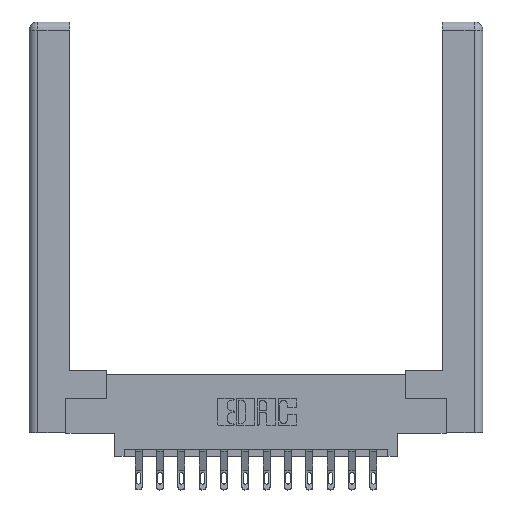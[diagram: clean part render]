
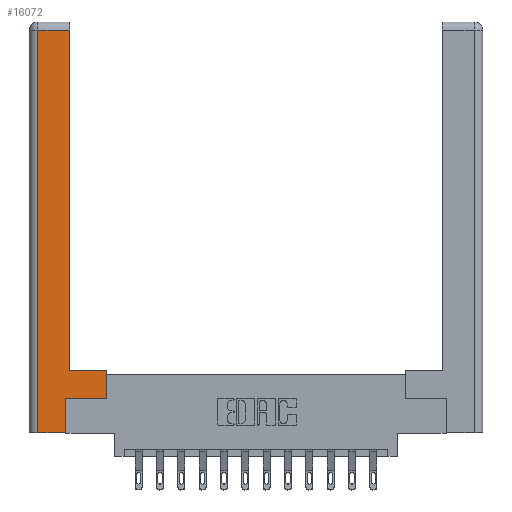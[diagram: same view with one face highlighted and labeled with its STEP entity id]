
A CAD part, top view. The second image highlights one B-rep face of the part: STEP entity #16072.
In plain terms, the highlighted planar face has unit normal (0, 0, 1).
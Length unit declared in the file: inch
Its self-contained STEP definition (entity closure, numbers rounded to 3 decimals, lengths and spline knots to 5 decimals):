
#4 = VERTEX_POINT ( 'NONE', #5458 ) ;
#204 = CARTESIAN_POINT ( 'NONE',  ( 0.0615, 0., 0. ) ) ;
#769 = EDGE_CURVE ( 'NONE', #12303, #15962, #13163, .T. ) ;
#890 = CARTESIAN_POINT ( 'NONE',  ( 0., 0., 0. ) ) ;
#1035 = VECTOR ( 'NONE', #10809, 39.37008 ) ;
#1246 = VECTOR ( 'NONE', #10216, 39.37008 ) ;
#1797 = CARTESIAN_POINT ( 'NONE',  ( 0.295, 2.94, 0. ) ) ;
#2032 = DIRECTION ( 'NONE',  ( 1., 0., 0. ) ) ;
#2476 = LINE ( 'NONE', #3857, #11309 ) ;
#3183 = ORIENTED_EDGE ( 'NONE', *, *, #4606, .T. ) ;
#3334 = ORIENTED_EDGE ( 'NONE', *, *, #7409, .T. ) ;
#3857 = CARTESIAN_POINT ( 'NONE',  ( 0.0615, 2.94, 0. ) ) ;
#3970 = CARTESIAN_POINT ( 'NONE',  ( 0.0615, 0., 0. ) ) ;
#4220 = VERTEX_POINT ( 'NONE', #6831 ) ;
#4551 = LINE ( 'NONE', #5077, #1246 ) ;
#4606 = EDGE_CURVE ( 'NONE', #12475, #7044, #2476, .T. ) ;
#4971 = DIRECTION ( 'NONE',  ( -1., 0., 0. ) ) ;
#5054 = CARTESIAN_POINT ( 'NONE',  ( 0.0615, 2.94, 0. ) ) ;
#5077 = CARTESIAN_POINT ( 'NONE',  ( 0.565, 0.45, 0. ) ) ;
#5188 = DIRECTION ( 'NONE',  ( 0., -1., 0. ) ) ;
#5458 = CARTESIAN_POINT ( 'NONE',  ( 0.565, 0.245, 0. ) ) ;
#5678 = AXIS2_PLACEMENT_3D ( 'NONE', #890, #9461, #12070 ) ;
#5933 = EDGE_CURVE ( 'NONE', #4220, #4, #11906, .T. ) ;
#6303 = CARTESIAN_POINT ( 'NONE',  ( 0.295, 0.45, 0. ) ) ;
#6445 = EDGE_CURVE ( 'NONE', #15962, #4220, #7293, .T. ) ;
#6590 = EDGE_LOOP ( 'NONE', ( #13713, #3183, #12075, #7782, #12550, #9775, #11407, #3334 ) ) ;
#6817 = VECTOR ( 'NONE', #2032, 39.37008 ) ;
#6831 = CARTESIAN_POINT ( 'NONE',  ( 0.265, 0.245, 0. ) ) ;
#6881 = CARTESIAN_POINT ( 'NONE',  ( 0.565, 0.45, 0. ) ) ;
#7044 = VERTEX_POINT ( 'NONE', #5054 ) ;
#7067 = PLANE ( 'NONE',  #5678 ) ;
#7175 = CARTESIAN_POINT ( 'NONE',  ( 0.295, 3., 0. ) ) ;
#7215 = VERTEX_POINT ( 'NONE', #8296 ) ;
#7276 = EDGE_CURVE ( 'NONE', #7215, #12475, #15420, .T. ) ;
#7293 = LINE ( 'NONE', #9532, #1035 ) ;
#7409 = EDGE_CURVE ( 'NONE', #12609, #7215, #15790, .T. ) ;
#7497 = LINE ( 'NONE', #204, #13440 ) ;
#7782 = ORIENTED_EDGE ( 'NONE', *, *, #769, .T. ) ;
#8262 = CARTESIAN_POINT ( 'NONE',  ( 0.265, 0., 0. ) ) ;
#8272 = VECTOR ( 'NONE', #8462, 39.37008 ) ;
#8296 = CARTESIAN_POINT ( 'NONE',  ( 0.295, 0.45, 0. ) ) ;
#8462 = DIRECTION ( 'NONE',  ( 0., 1., 0. ) ) ;
#8713 = VECTOR ( 'NONE', #12404, 39.37008 ) ;
#9461 = DIRECTION ( 'NONE',  ( 0., 0., -1. ) ) ;
#9532 = CARTESIAN_POINT ( 'NONE',  ( 0.265, 0.245, 0. ) ) ;
#9775 = ORIENTED_EDGE ( 'NONE', *, *, #5933, .T. ) ;
#10216 = DIRECTION ( 'NONE',  ( 0., 1., 0. ) ) ;
#10809 = DIRECTION ( 'NONE',  ( 0., 1., 0. ) ) ;
#11309 = VECTOR ( 'NONE', #11817, 39.37008 ) ;
#11407 = ORIENTED_EDGE ( 'NONE', *, *, #14374, .T. ) ;
#11817 = DIRECTION ( 'NONE',  ( -1., 0., 0. ) ) ;
#11906 = LINE ( 'NONE', #13725, #8713 ) ;
#12070 = DIRECTION ( 'NONE',  ( -1., 0., 0. ) ) ;
#12075 = ORIENTED_EDGE ( 'NONE', *, *, #14395, .T. ) ;
#12303 = VERTEX_POINT ( 'NONE', #3970 ) ;
#12404 = DIRECTION ( 'NONE',  ( 1., 0., 0. ) ) ;
#12429 = VECTOR ( 'NONE', #4971, 39.37008 ) ;
#12475 = VERTEX_POINT ( 'NONE', #1797 ) ;
#12550 = ORIENTED_EDGE ( 'NONE', *, *, #6445, .T. ) ;
#12609 = VERTEX_POINT ( 'NONE', #6881 ) ;
#12764 = FACE_OUTER_BOUND ( 'NONE', #6590, .T. ) ;
#13163 = LINE ( 'NONE', #8262, #6817 ) ;
#13440 = VECTOR ( 'NONE', #5188, 39.37008 ) ;
#13713 = ORIENTED_EDGE ( 'NONE', *, *, #7276, .T. ) ;
#13725 = CARTESIAN_POINT ( 'NONE',  ( 0.565, 0.245, 0. ) ) ;
#14005 = CARTESIAN_POINT ( 'NONE',  ( 0.265, 0., 0. ) ) ;
#14374 = EDGE_CURVE ( 'NONE', #4, #12609, #4551, .T. ) ;
#14395 = EDGE_CURVE ( 'NONE', #7044, #12303, #7497, .T. ) ;
#15420 = LINE ( 'NONE', #7175, #8272 ) ;
#15790 = LINE ( 'NONE', #6303, #12429 ) ;
#15962 = VERTEX_POINT ( 'NONE', #14005 ) ;
#16072 = ADVANCED_FACE ( 'NONE', ( #12764 ), #7067, .F. ) ;
